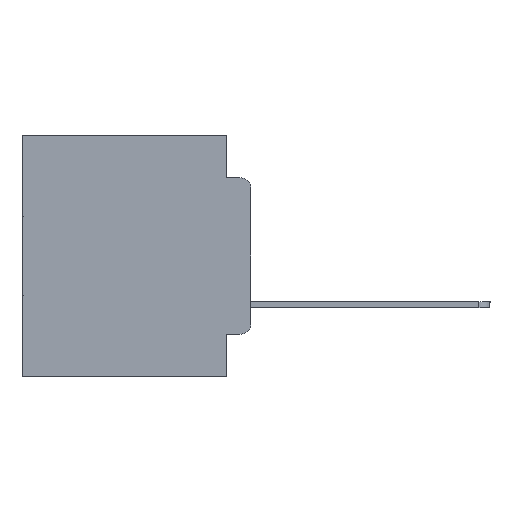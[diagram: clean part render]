
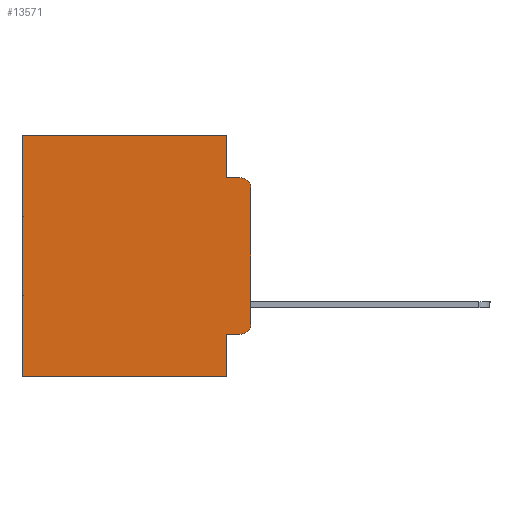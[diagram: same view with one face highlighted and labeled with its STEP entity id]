
A CAD part, left-side view. The second image highlights one B-rep face of the part: STEP entity #13571.
In plain terms, the highlighted planar face has unit normal (-1, 0, 0).
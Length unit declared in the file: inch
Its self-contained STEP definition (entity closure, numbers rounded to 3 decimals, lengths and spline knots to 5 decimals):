
#736 = VERTEX_POINT ( 'NONE', #2183 ) ;
#788 = CARTESIAN_POINT ( 'NONE',  ( 0.298, 0.02, -0.1085 ) ) ;
#1271 = ORIENTED_EDGE ( 'NONE', *, *, #12742, .F. ) ;
#2183 = CARTESIAN_POINT ( 'NONE',  ( 0.298, 0.051, 0. ) ) ;
#2366 = DIRECTION ( 'NONE',  ( 0., 0., -1. ) ) ;
#2681 = CARTESIAN_POINT ( 'NONE',  ( 0.298, 0.02, -0.0885 ) ) ;
#3700 = CARTESIAN_POINT ( 'NONE',  ( 0.298, 0.02, -0.3915 ) ) ;
#4041 = EDGE_CURVE ( 'NONE', #24285, #17413, #17681, .T. ) ;
#4049 = DIRECTION ( 'NONE',  ( 0., 0., -1. ) ) ;
#4200 = LINE ( 'NONE', #16053, #9901 ) ;
#4393 = CARTESIAN_POINT ( 'NONE',  ( 0.298, 0., 0. ) ) ;
#4466 = CIRCLE ( 'NONE', #8879, 0.02 ) ;
#4552 = VERTEX_POINT ( 'NONE', #11293 ) ;
#4862 = EDGE_CURVE ( 'NONE', #5984, #5725, #17984, .T. ) ;
#5317 = ORIENTED_EDGE ( 'NONE', *, *, #30087, .F. ) ;
#5525 = LINE ( 'NONE', #14913, #16428 ) ;
#5623 = LINE ( 'NONE', #19815, #27594 ) ;
#5725 = VERTEX_POINT ( 'NONE', #2681 ) ;
#5815 = DIRECTION ( 'NONE',  ( 0., 1., 0. ) ) ;
#5984 = VERTEX_POINT ( 'NONE', #29402 ) ;
#6015 = CARTESIAN_POINT ( 'NONE',  ( 0.298, 0.051, -0.4115 ) ) ;
#6242 = VECTOR ( 'NONE', #11490, 39.37008 ) ;
#6405 = ORIENTED_EDGE ( 'NONE', *, *, #14135, .T. ) ;
#6454 = EDGE_CURVE ( 'NONE', #29261, #24285, #16603, .T. ) ;
#6706 = PLANE ( 'NONE',  #13888 ) ;
#7818 = LINE ( 'NONE', #28712, #10786 ) ;
#8388 = CARTESIAN_POINT ( 'NONE',  ( 0.298, 0.02, -0.4115 ) ) ;
#8879 = AXIS2_PLACEMENT_3D ( 'NONE', #3700, #13071, #24120 ) ;
#9137 = VECTOR ( 'NONE', #19712, 39.37008 ) ;
#9901 = VECTOR ( 'NONE', #4049, 39.37008 ) ;
#9902 = LINE ( 'NONE', #19347, #20350 ) ;
#10786 = VECTOR ( 'NONE', #19568, 39.37008 ) ;
#11293 = CARTESIAN_POINT ( 'NONE',  ( 0.298, 0.473, 0. ) ) ;
#11490 = DIRECTION ( 'NONE',  ( 0., 0., -1. ) ) ;
#12742 = EDGE_CURVE ( 'NONE', #736, #27356, #4200, .T. ) ;
#12875 = CARTESIAN_POINT ( 'NONE',  ( 0.298, 0., -0.5 ) ) ;
#13071 = DIRECTION ( 'NONE',  ( -1., 0., 0. ) ) ;
#13136 = VERTEX_POINT ( 'NONE', #27936 ) ;
#13571 = ADVANCED_FACE ( 'NONE', ( #27721 ), #6706, .F. ) ;
#13770 = DIRECTION ( 'NONE',  ( 1., 0., 0. ) ) ;
#13808 = EDGE_CURVE ( 'NONE', #29261, #25332, #9902, .T. ) ;
#13888 = AXIS2_PLACEMENT_3D ( 'NONE', #4393, #13770, #2366 ) ;
#14135 = EDGE_CURVE ( 'NONE', #736, #4552, #5525, .T. ) ;
#14683 = DIRECTION ( 'NONE',  ( 0., -1., 0. ) ) ;
#14913 = CARTESIAN_POINT ( 'NONE',  ( 0.298, 0., 0. ) ) ;
#14942 = ORIENTED_EDGE ( 'NONE', *, *, #23892, .T. ) ;
#14983 = ORIENTED_EDGE ( 'NONE', *, *, #4862, .T. ) ;
#15203 = ORIENTED_EDGE ( 'NONE', *, *, #6454, .F. ) ;
#16053 = CARTESIAN_POINT ( 'NONE',  ( 0.298, 0.051, 0. ) ) ;
#16428 = VECTOR ( 'NONE', #5815, 39.37008 ) ;
#16510 = ORIENTED_EDGE ( 'NONE', *, *, #13808, .T. ) ;
#16603 = LINE ( 'NONE', #26031, #6242 ) ;
#17413 = VERTEX_POINT ( 'NONE', #17825 ) ;
#17615 = CARTESIAN_POINT ( 'NONE',  ( 0.298, 0.051, -0.0885 ) ) ;
#17681 = LINE ( 'NONE', #12875, #9137 ) ;
#17825 = CARTESIAN_POINT ( 'NONE',  ( 0.298, 0.473, -0.5 ) ) ;
#17984 = CIRCLE ( 'NONE', #27377, 0.02 ) ;
#18916 = LINE ( 'NONE', #28359, #24833 ) ;
#19347 = CARTESIAN_POINT ( 'NONE',  ( 0.298, 0.051, -0.4115 ) ) ;
#19537 = ORIENTED_EDGE ( 'NONE', *, *, #4041, .F. ) ;
#19568 = DIRECTION ( 'NONE',  ( 0., -1., 0. ) ) ;
#19712 = DIRECTION ( 'NONE',  ( 0., 1., 0. ) ) ;
#19815 = CARTESIAN_POINT ( 'NONE',  ( 0.298, 0., 0. ) ) ;
#20046 = DIRECTION ( 'NONE',  ( -1., 0., 0. ) ) ;
#20350 = VECTOR ( 'NONE', #14683, 39.37008 ) ;
#23074 = DIRECTION ( 'NONE',  ( 0., 0., -1. ) ) ;
#23799 = EDGE_LOOP ( 'NONE', ( #5317, #14983, #25005, #1271, #6405, #14942, #19537, #15203, #16510, #27301 ) ) ;
#23892 = EDGE_CURVE ( 'NONE', #4552, #17413, #18916, .T. ) ;
#24108 = DIRECTION ( 'NONE',  ( 0., 0., -1. ) ) ;
#24120 = DIRECTION ( 'NONE',  ( 0., 0., -1. ) ) ;
#24285 = VERTEX_POINT ( 'NONE', #28754 ) ;
#24833 = VECTOR ( 'NONE', #23074, 39.37008 ) ;
#25005 = ORIENTED_EDGE ( 'NONE', *, *, #29426, .F. ) ;
#25332 = VERTEX_POINT ( 'NONE', #8388 ) ;
#26031 = CARTESIAN_POINT ( 'NONE',  ( 0.298, 0.051, 0. ) ) ;
#27062 = DIRECTION ( 'NONE',  ( 0., 0., -1. ) ) ;
#27301 = ORIENTED_EDGE ( 'NONE', *, *, #29310, .T. ) ;
#27356 = VERTEX_POINT ( 'NONE', #17615 ) ;
#27377 = AXIS2_PLACEMENT_3D ( 'NONE', #788, #20046, #24108 ) ;
#27594 = VECTOR ( 'NONE', #27062, 39.37008 ) ;
#27721 = FACE_OUTER_BOUND ( 'NONE', #23799, .T. ) ;
#27936 = CARTESIAN_POINT ( 'NONE',  ( 0.298, 0., -0.3915 ) ) ;
#28359 = CARTESIAN_POINT ( 'NONE',  ( 0.298, 0.473, 0. ) ) ;
#28712 = CARTESIAN_POINT ( 'NONE',  ( 0.298, 0.051, -0.0885 ) ) ;
#28754 = CARTESIAN_POINT ( 'NONE',  ( 0.298, 0.051, -0.5 ) ) ;
#29261 = VERTEX_POINT ( 'NONE', #6015 ) ;
#29310 = EDGE_CURVE ( 'NONE', #25332, #13136, #4466, .T. ) ;
#29402 = CARTESIAN_POINT ( 'NONE',  ( 0.298, 0., -0.1085 ) ) ;
#29426 = EDGE_CURVE ( 'NONE', #27356, #5725, #7818, .T. ) ;
#30087 = EDGE_CURVE ( 'NONE', #5984, #13136, #5623, .T. ) ;
